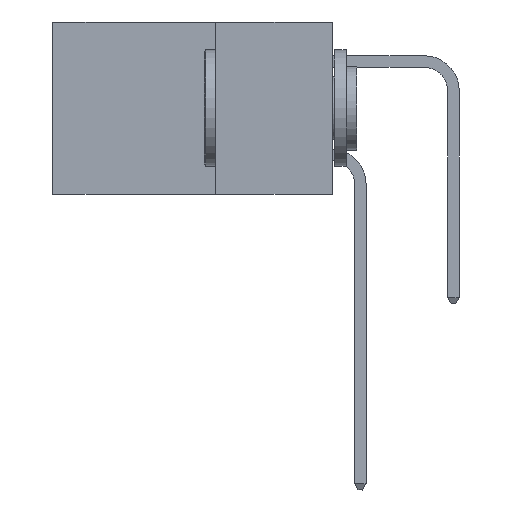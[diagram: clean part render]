
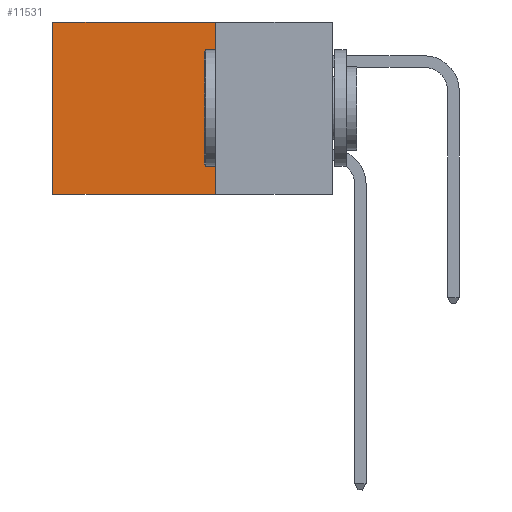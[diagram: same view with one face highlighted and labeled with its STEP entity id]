
A CAD part, left-side view. The second image highlights one B-rep face of the part: STEP entity #11531.
In plain terms, the highlighted planar face has unit normal (-1, 0, 0).
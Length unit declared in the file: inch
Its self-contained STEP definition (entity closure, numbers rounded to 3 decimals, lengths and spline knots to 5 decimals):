
#14 = CARTESIAN_POINT ( 'NONE',  ( 0.2615, 0.25, -0.37 ) ) ;
#734 = VERTEX_POINT ( 'NONE', #17781 ) ;
#1405 = LINE ( 'NONE', #7467, #12798 ) ;
#2363 = VECTOR ( 'NONE', #16520, 39.37008 ) ;
#2960 = CARTESIAN_POINT ( 'NONE',  ( 0.2615, 0.25, -0.37 ) ) ;
#3007 = DIRECTION ( 'NONE',  ( 1., 0., 0. ) ) ;
#3399 = CARTESIAN_POINT ( 'NONE',  ( 0.2615, 0.6, -0.37 ) ) ;
#4314 = EDGE_CURVE ( 'NONE', #734, #13085, #1405, .T. ) ;
#5289 = DIRECTION ( 'NONE',  ( 0., 1., 0. ) ) ;
#5559 = LINE ( 'NONE', #2960, #2363 ) ;
#5829 = ORIENTED_EDGE ( 'NONE', *, *, #4314, .T. ) ;
#7355 = CARTESIAN_POINT ( 'NONE',  ( 0.2615, 0.25, -0.37 ) ) ;
#7467 = CARTESIAN_POINT ( 'NONE',  ( 0.2615, 0.25, 0. ) ) ;
#9055 = ORIENTED_EDGE ( 'NONE', *, *, #23875, .F. ) ;
#9741 = AXIS2_PLACEMENT_3D ( 'NONE', #7355, #3007, #9800 ) ;
#9800 = DIRECTION ( 'NONE',  ( 0., 0., -1. ) ) ;
#11422 = EDGE_CURVE ( 'NONE', #18887, #25270, #11674, .T. ) ;
#11531 = ADVANCED_FACE ( 'NONE', ( #27108 ), #23057, .F. ) ;
#11674 = LINE ( 'NONE', #14, #15838 ) ;
#12145 = ORIENTED_EDGE ( 'NONE', *, *, #11422, .F. ) ;
#12798 = VECTOR ( 'NONE', #5289, 39.37008 ) ;
#13085 = VERTEX_POINT ( 'NONE', #25495 ) ;
#13220 = CARTESIAN_POINT ( 'NONE',  ( 0.2615, 0.25, -0.37 ) ) ;
#13262 = DIRECTION ( 'NONE',  ( 0., 1., 0. ) ) ;
#13519 = EDGE_LOOP ( 'NONE', ( #24507, #12145, #9055, #5829 ) ) ;
#15461 = CARTESIAN_POINT ( 'NONE',  ( 0.2615, 0.6, -0.37 ) ) ;
#15838 = VECTOR ( 'NONE', #13262, 39.37008 ) ;
#16520 = DIRECTION ( 'NONE',  ( 0., 0., -1. ) ) ;
#17006 = EDGE_CURVE ( 'NONE', #13085, #25270, #19803, .T. ) ;
#17781 = CARTESIAN_POINT ( 'NONE',  ( 0.2615, 0.25, 0. ) ) ;
#18887 = VERTEX_POINT ( 'NONE', #13220 ) ;
#19803 = LINE ( 'NONE', #15461, #23841 ) ;
#22111 = DIRECTION ( 'NONE',  ( 0., 0., -1. ) ) ;
#23057 = PLANE ( 'NONE',  #9741 ) ;
#23841 = VECTOR ( 'NONE', #22111, 39.37008 ) ;
#23875 = EDGE_CURVE ( 'NONE', #734, #18887, #5559, .T. ) ;
#24507 = ORIENTED_EDGE ( 'NONE', *, *, #17006, .T. ) ;
#25270 = VERTEX_POINT ( 'NONE', #3399 ) ;
#25495 = CARTESIAN_POINT ( 'NONE',  ( 0.2615, 0.6, 0. ) ) ;
#27108 = FACE_OUTER_BOUND ( 'NONE', #13519, .T. ) ;
